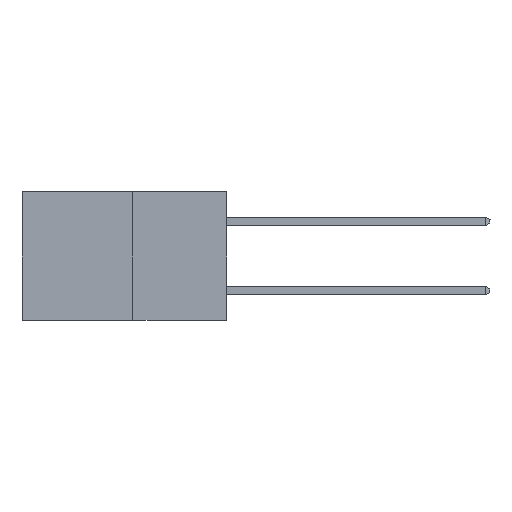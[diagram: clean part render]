
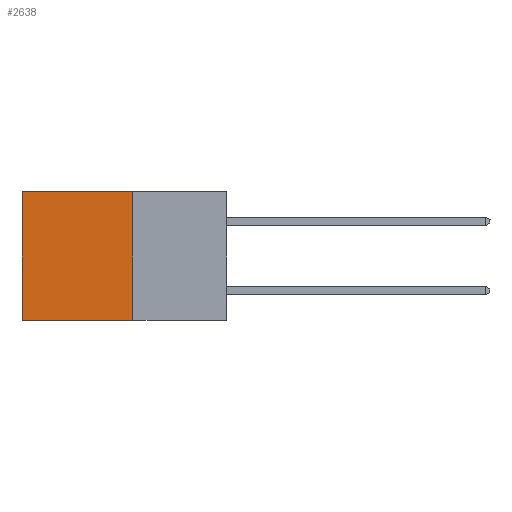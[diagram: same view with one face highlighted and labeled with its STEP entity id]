
A CAD part, left-side view. The second image highlights one B-rep face of the part: STEP entity #2638.
In plain terms, the highlighted planar face has unit normal (-1, 0, 0).
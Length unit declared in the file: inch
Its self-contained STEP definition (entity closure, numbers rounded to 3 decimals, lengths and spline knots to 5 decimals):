
#2367 = LINE ( 'NONE', #13441, #22585 ) ;
#2638 = ADVANCED_FACE ( 'NONE', ( #14416 ), #17602, .F. ) ;
#2795 = AXIS2_PLACEMENT_3D ( 'NONE', #17982, #2932, #14531 ) ;
#2932 = DIRECTION ( 'NONE',  ( 1., 0., 0. ) ) ;
#3742 = CARTESIAN_POINT ( 'NONE',  ( 0.277, 0.27, 0. ) ) ;
#6386 = VERTEX_POINT ( 'NONE', #17619 ) ;
#7300 = ORIENTED_EDGE ( 'NONE', *, *, #16025, .T. ) ;
#7845 = VERTEX_POINT ( 'NONE', #8440 ) ;
#8044 = LINE ( 'NONE', #17103, #18148 ) ;
#8440 = CARTESIAN_POINT ( 'NONE',  ( 0.277, 0.27, -0.37 ) ) ;
#8993 = VERTEX_POINT ( 'NONE', #17653 ) ;
#9036 = CARTESIAN_POINT ( 'NONE',  ( 0.277, 0.59, 0. ) ) ;
#9355 = EDGE_LOOP ( 'NONE', ( #7300, #23486, #20199, #25590 ) ) ;
#11451 = VECTOR ( 'NONE', #16212, 39.37008 ) ;
#11542 = EDGE_CURVE ( 'NONE', #7845, #6386, #22128, .T. ) ;
#11880 = VERTEX_POINT ( 'NONE', #9036 ) ;
#13441 = CARTESIAN_POINT ( 'NONE',  ( 0.277, 0.27, -0.37 ) ) ;
#14416 = FACE_OUTER_BOUND ( 'NONE', #9355, .T. ) ;
#14531 = DIRECTION ( 'NONE',  ( 0., 0., -1. ) ) ;
#14931 = VECTOR ( 'NONE', #21923, 39.37008 ) ;
#16025 = EDGE_CURVE ( 'NONE', #11880, #6386, #8044, .T. ) ;
#16212 = DIRECTION ( 'NONE',  ( 0., 1., 0. ) ) ;
#17103 = CARTESIAN_POINT ( 'NONE',  ( 0.277, 0.59, -0.37 ) ) ;
#17602 = PLANE ( 'NONE',  #2795 ) ;
#17619 = CARTESIAN_POINT ( 'NONE',  ( 0.277, 0.59, -0.37 ) ) ;
#17653 = CARTESIAN_POINT ( 'NONE',  ( 0.277, 0.27, 0. ) ) ;
#17982 = CARTESIAN_POINT ( 'NONE',  ( 0.277, 0.27, -0.37 ) ) ;
#18148 = VECTOR ( 'NONE', #19124, 39.37008 ) ;
#18764 = EDGE_CURVE ( 'NONE', #8993, #7845, #2367, .T. ) ;
#19124 = DIRECTION ( 'NONE',  ( 0., 0., -1. ) ) ;
#20199 = ORIENTED_EDGE ( 'NONE', *, *, #18764, .F. ) ;
#20256 = LINE ( 'NONE', #3742, #14931 ) ;
#21923 = DIRECTION ( 'NONE',  ( 0., 1., 0. ) ) ;
#21945 = EDGE_CURVE ( 'NONE', #8993, #11880, #20256, .T. ) ;
#22128 = LINE ( 'NONE', #24164, #11451 ) ;
#22585 = VECTOR ( 'NONE', #25392, 39.37008 ) ;
#23486 = ORIENTED_EDGE ( 'NONE', *, *, #11542, .F. ) ;
#24164 = CARTESIAN_POINT ( 'NONE',  ( 0.277, 0.27, -0.37 ) ) ;
#25392 = DIRECTION ( 'NONE',  ( 0., 0., -1. ) ) ;
#25590 = ORIENTED_EDGE ( 'NONE', *, *, #21945, .T. ) ;
